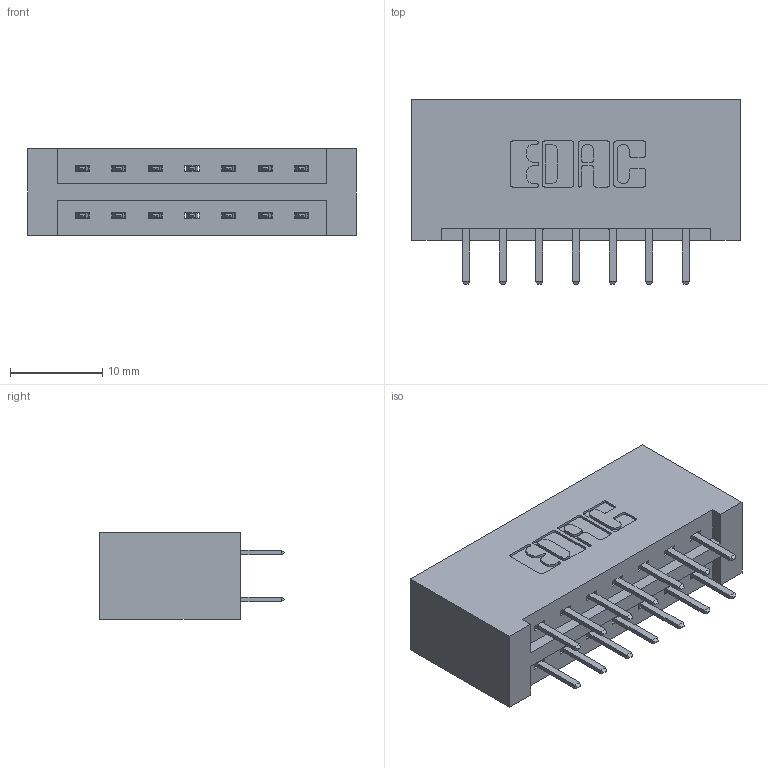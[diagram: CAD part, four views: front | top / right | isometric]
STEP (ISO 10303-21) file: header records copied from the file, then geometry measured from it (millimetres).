
FILE_DESCRIPTION (( 'STEP AP203' ), '1' );
FILE_NAME ('387-014-520-201.STEP', '2018-09-11T01:16:05', ( '' ), ( '' ), 'SwSTEP 2.0', 'SolidWorks 2016', '' );
FILE_SCHEMA (( 'CONFIG_CONTROL_DESIGN' ));
Length unit declared in the file: inch
Products named in the file (3): 337 Part_No Mounting Lugs; 345-292-001_345-293-120; 387-014-520-201
Assembly tree (15 placements, depth 2):
  387-014-520-201
    337 Part_No Mounting Lugs
    345-292-001_345-293-120  x14
Bounding box: 35.61 x 20.02 x 9.4 mm (x, y, z)
Volume: 4041.6 mm3; surface area: 4267.7 mm2
Topology: 15 solids, 15 shells, 918 faces, 2653 edges, 1730 vertices
Faces by surface type: plane 626, cylinder 292
Entity records: 9791 total; most frequent: CARTESIAN_POINT 1690, ORIENTED_EDGE 1614, DIRECTION 1483, EDGE_CURVE 807, LINE 683, VECTOR 683, VERTEX_POINT 534, AXIS2_PLACEMENT_3D 400
